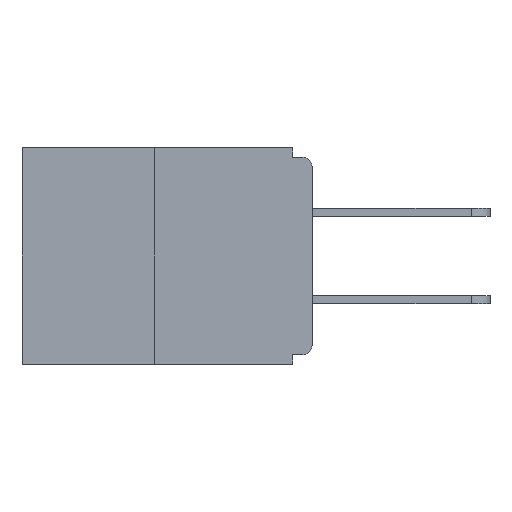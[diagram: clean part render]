
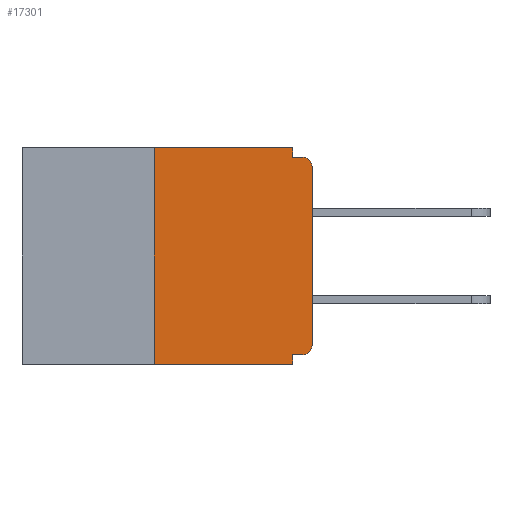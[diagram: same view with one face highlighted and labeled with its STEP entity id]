
A CAD part, left-side view. The second image highlights one B-rep face of the part: STEP entity #17301.
In plain terms, the highlighted planar face has unit normal (-1, 0, 0).
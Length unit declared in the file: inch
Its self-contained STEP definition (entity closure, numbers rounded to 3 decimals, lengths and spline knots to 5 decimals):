
#141 = CARTESIAN_POINT ( 'NONE',  ( 0., 0.015, -0.328 ) ) ;
#202 = DIRECTION ( 'NONE',  ( 0., 0., -1. ) ) ;
#387 = EDGE_LOOP ( 'NONE', ( #20647, #5497, #18754, #1826, #4495, #22314, #10986, #11658, #4504, #7663 ) ) ;
#1090 = CARTESIAN_POINT ( 'NONE',  ( 0., 0.015, -0.015 ) ) ;
#1379 = VECTOR ( 'NONE', #6203, 39.37008 ) ;
#1608 = CARTESIAN_POINT ( 'NONE',  ( 0., 0.031, -0.015 ) ) ;
#1684 = EDGE_CURVE ( 'NONE', #11121, #4698, #14064, .T. ) ;
#1826 = ORIENTED_EDGE ( 'NONE', *, *, #7278, .F. ) ;
#1868 = CARTESIAN_POINT ( 'NONE',  ( 0., 0., -0.328 ) ) ;
#1928 = CARTESIAN_POINT ( 'NONE',  ( 0., 0.031, -0.343 ) ) ;
#1977 = VERTEX_POINT ( 'NONE', #17725 ) ;
#2755 = VERTEX_POINT ( 'NONE', #1090 ) ;
#3718 = DIRECTION ( 'NONE',  ( 0., 0., 1. ) ) ;
#3753 = CIRCLE ( 'NONE', #13579, 0.015 ) ;
#3838 = VERTEX_POINT ( 'NONE', #13101 ) ;
#4377 = EDGE_CURVE ( 'NONE', #12475, #2755, #13388, .T. ) ;
#4495 = ORIENTED_EDGE ( 'NONE', *, *, #19931, .F. ) ;
#4504 = ORIENTED_EDGE ( 'NONE', *, *, #4377, .F. ) ;
#4617 = CARTESIAN_POINT ( 'NONE',  ( 0., 0.25, 0. ) ) ;
#4698 = VERTEX_POINT ( 'NONE', #18650 ) ;
#5362 = CARTESIAN_POINT ( 'NONE',  ( 0., 0., -0.015 ) ) ;
#5497 = ORIENTED_EDGE ( 'NONE', *, *, #8985, .F. ) ;
#5691 = VECTOR ( 'NONE', #20875, 39.37008 ) ;
#5845 = DIRECTION ( 'NONE',  ( 0., 0., -1. ) ) ;
#6203 = DIRECTION ( 'NONE',  ( 0., 0., 1. ) ) ;
#6258 = VERTEX_POINT ( 'NONE', #17946 ) ;
#6299 = DIRECTION ( 'NONE',  ( 0., -1., 0. ) ) ;
#6320 = VERTEX_POINT ( 'NONE', #19977 ) ;
#6978 = DIRECTION ( 'NONE',  ( 0., 0., -1. ) ) ;
#7171 = DIRECTION ( 'NONE',  ( 0., -1., 0. ) ) ;
#7253 = LINE ( 'NONE', #19969, #21893 ) ;
#7278 = EDGE_CURVE ( 'NONE', #11085, #6320, #14476, .T. ) ;
#7584 = AXIS2_PLACEMENT_3D ( 'NONE', #15228, #18702, #11546 ) ;
#7663 = ORIENTED_EDGE ( 'NONE', *, *, #17110, .F. ) ;
#8508 = VECTOR ( 'NONE', #17508, 39.37008 ) ;
#8985 = EDGE_CURVE ( 'NONE', #3838, #11121, #9765, .T. ) ;
#9213 = CARTESIAN_POINT ( 'NONE',  ( 0., 0.031, 0. ) ) ;
#9324 = VECTOR ( 'NONE', #7171, 39.37008 ) ;
#9765 = LINE ( 'NONE', #4617, #1379 ) ;
#10481 = CARTESIAN_POINT ( 'NONE',  ( 0., 0.015, -0.03 ) ) ;
#10526 = PLANE ( 'NONE',  #18897 ) ;
#10576 = EDGE_CURVE ( 'NONE', #6258, #1977, #11293, .T. ) ;
#10607 = CARTESIAN_POINT ( 'NONE',  ( 0., 0.46, 0. ) ) ;
#10802 = LINE ( 'NONE', #1868, #5691 ) ;
#10986 = ORIENTED_EDGE ( 'NONE', *, *, #10576, .T. ) ;
#11031 = EDGE_CURVE ( 'NONE', #3838, #6320, #7253, .T. ) ;
#11085 = VERTEX_POINT ( 'NONE', #11625 ) ;
#11121 = VERTEX_POINT ( 'NONE', #22055 ) ;
#11293 = LINE ( 'NONE', #15600, #19976 ) ;
#11488 = FACE_OUTER_BOUND ( 'NONE', #387, .T. ) ;
#11546 = DIRECTION ( 'NONE',  ( 0., 0., -1. ) ) ;
#11625 = CARTESIAN_POINT ( 'NONE',  ( 0., 0.031, -0.328 ) ) ;
#11658 = ORIENTED_EDGE ( 'NONE', *, *, #20876, .T. ) ;
#12475 = VERTEX_POINT ( 'NONE', #1608 ) ;
#12737 = VECTOR ( 'NONE', #6299, 39.37008 ) ;
#13101 = CARTESIAN_POINT ( 'NONE',  ( 0., 0.25, -0.343 ) ) ;
#13144 = LINE ( 'NONE', #9213, #20732 ) ;
#13388 = LINE ( 'NONE', #5362, #9324 ) ;
#13579 = AXIS2_PLACEMENT_3D ( 'NONE', #10481, #17321, #6978 ) ;
#13661 = EDGE_CURVE ( 'NONE', #19972, #6258, #14389, .T. ) ;
#14064 = LINE ( 'NONE', #15149, #12737 ) ;
#14389 = CIRCLE ( 'NONE', #7584, 0.015 ) ;
#14476 = LINE ( 'NONE', #1928, #8508 ) ;
#14559 = DIRECTION ( 'NONE',  ( 0., -1., 0. ) ) ;
#15149 = CARTESIAN_POINT ( 'NONE',  ( 0., 0.46, 0. ) ) ;
#15228 = CARTESIAN_POINT ( 'NONE',  ( 0., 0.015, -0.313 ) ) ;
#15600 = CARTESIAN_POINT ( 'NONE',  ( 0., 0., 0. ) ) ;
#17110 = EDGE_CURVE ( 'NONE', #4698, #12475, #13144, .T. ) ;
#17301 = ADVANCED_FACE ( 'NONE', ( #11488 ), #10526, .F. ) ;
#17321 = DIRECTION ( 'NONE',  ( -1., 0., 0. ) ) ;
#17508 = DIRECTION ( 'NONE',  ( 0., 0., -1. ) ) ;
#17725 = CARTESIAN_POINT ( 'NONE',  ( 0., 0., -0.03 ) ) ;
#17946 = CARTESIAN_POINT ( 'NONE',  ( 0., 0., -0.313 ) ) ;
#18650 = CARTESIAN_POINT ( 'NONE',  ( 0., 0.031, 0. ) ) ;
#18702 = DIRECTION ( 'NONE',  ( -1., 0., 0. ) ) ;
#18754 = ORIENTED_EDGE ( 'NONE', *, *, #11031, .T. ) ;
#18897 = AXIS2_PLACEMENT_3D ( 'NONE', #10607, #19112, #202 ) ;
#19112 = DIRECTION ( 'NONE',  ( 1., 0., 0. ) ) ;
#19931 = EDGE_CURVE ( 'NONE', #19972, #11085, #10802, .T. ) ;
#19969 = CARTESIAN_POINT ( 'NONE',  ( 0., 0.46, -0.343 ) ) ;
#19972 = VERTEX_POINT ( 'NONE', #141 ) ;
#19976 = VECTOR ( 'NONE', #3718, 39.37008 ) ;
#19977 = CARTESIAN_POINT ( 'NONE',  ( 0., 0.031, -0.343 ) ) ;
#20647 = ORIENTED_EDGE ( 'NONE', *, *, #1684, .F. ) ;
#20732 = VECTOR ( 'NONE', #5845, 39.37008 ) ;
#20875 = DIRECTION ( 'NONE',  ( 0., 1., 0. ) ) ;
#20876 = EDGE_CURVE ( 'NONE', #1977, #2755, #3753, .T. ) ;
#21893 = VECTOR ( 'NONE', #14559, 39.37008 ) ;
#22055 = CARTESIAN_POINT ( 'NONE',  ( 0., 0.25, 0. ) ) ;
#22314 = ORIENTED_EDGE ( 'NONE', *, *, #13661, .T. ) ;
